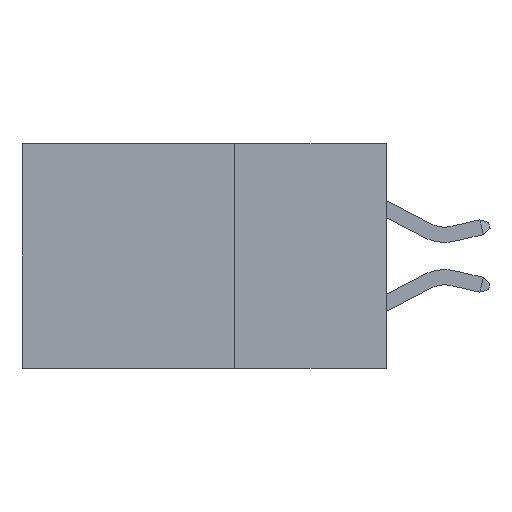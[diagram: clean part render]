
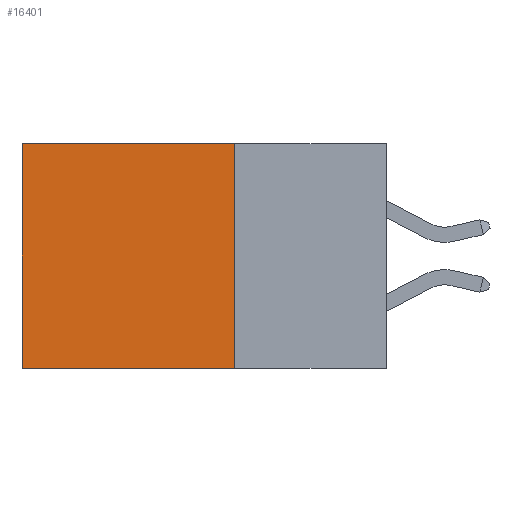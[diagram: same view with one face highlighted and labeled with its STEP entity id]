
A CAD part, left-side view. The second image highlights one B-rep face of the part: STEP entity #16401.
In plain terms, the highlighted planar face has unit normal (-1, 0, 0).
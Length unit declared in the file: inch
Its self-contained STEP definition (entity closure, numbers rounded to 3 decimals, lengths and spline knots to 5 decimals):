
#84 = DIRECTION ( 'NONE',  ( 0., 0., -1. ) ) ;
#208 = ORIENTED_EDGE ( 'NONE', *, *, #11704, .F. ) ;
#2570 = CARTESIAN_POINT ( 'NONE',  ( 0.298, 0.25, 0. ) ) ;
#4392 = LINE ( 'NONE', #27684, #15027 ) ;
#4847 = DIRECTION ( 'NONE',  ( 0., 1., 0. ) ) ;
#4995 = CARTESIAN_POINT ( 'NONE',  ( 0.298, 0.25, 0. ) ) ;
#6531 = CARTESIAN_POINT ( 'NONE',  ( 0.298, 0.25, -0.37 ) ) ;
#6923 = ORIENTED_EDGE ( 'NONE', *, *, #8769, .T. ) ;
#8538 = VECTOR ( 'NONE', #4847, 39.37008 ) ;
#8769 = EDGE_CURVE ( 'NONE', #12778, #14237, #4392, .T. ) ;
#10791 = EDGE_CURVE ( 'NONE', #24643, #12778, #20464, .T. ) ;
#11703 = DIRECTION ( 'NONE',  ( 0., 0., -1. ) ) ;
#11704 = EDGE_CURVE ( 'NONE', #20769, #14237, #26968, .T. ) ;
#11984 = ORIENTED_EDGE ( 'NONE', *, *, #22051, .F. ) ;
#12778 = VERTEX_POINT ( 'NONE', #22325 ) ;
#13272 = ORIENTED_EDGE ( 'NONE', *, *, #10791, .T. ) ;
#14237 = VERTEX_POINT ( 'NONE', #24783 ) ;
#14802 = CARTESIAN_POINT ( 'NONE',  ( 0.298, 0.25, -0.37 ) ) ;
#15027 = VECTOR ( 'NONE', #84, 39.37008 ) ;
#16401 = ADVANCED_FACE ( 'NONE', ( #28135 ), #22863, .F. ) ;
#20464 = LINE ( 'NONE', #2570, #8538 ) ;
#20769 = VERTEX_POINT ( 'NONE', #6531 ) ;
#22051 = EDGE_CURVE ( 'NONE', #24643, #20769, #23855, .T. ) ;
#22325 = CARTESIAN_POINT ( 'NONE',  ( 0.298, 0.6, 0. ) ) ;
#22711 = AXIS2_PLACEMENT_3D ( 'NONE', #24893, #25086, #11703 ) ;
#22863 = PLANE ( 'NONE',  #22711 ) ;
#23165 = VECTOR ( 'NONE', #25210, 39.37008 ) ;
#23762 = DIRECTION ( 'NONE',  ( 0., 1., 0. ) ) ;
#23855 = LINE ( 'NONE', #4995, #23165 ) ;
#24643 = VERTEX_POINT ( 'NONE', #25753 ) ;
#24783 = CARTESIAN_POINT ( 'NONE',  ( 0.298, 0.6, -0.37 ) ) ;
#24893 = CARTESIAN_POINT ( 'NONE',  ( 0.298, 0.25, 0. ) ) ;
#25086 = DIRECTION ( 'NONE',  ( 1., 0., 0. ) ) ;
#25210 = DIRECTION ( 'NONE',  ( 0., 0., -1. ) ) ;
#25384 = EDGE_LOOP ( 'NONE', ( #6923, #208, #11984, #13272 ) ) ;
#25753 = CARTESIAN_POINT ( 'NONE',  ( 0.298, 0.25, 0. ) ) ;
#26291 = VECTOR ( 'NONE', #23762, 39.37008 ) ;
#26968 = LINE ( 'NONE', #14802, #26291 ) ;
#27684 = CARTESIAN_POINT ( 'NONE',  ( 0.298, 0.6, 0. ) ) ;
#28135 = FACE_OUTER_BOUND ( 'NONE', #25384, .T. ) ;
